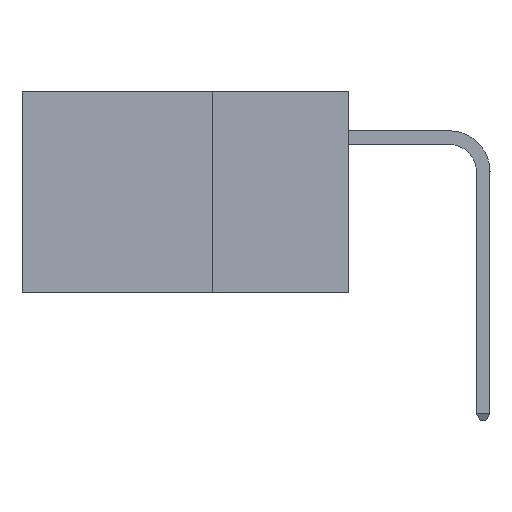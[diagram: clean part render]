
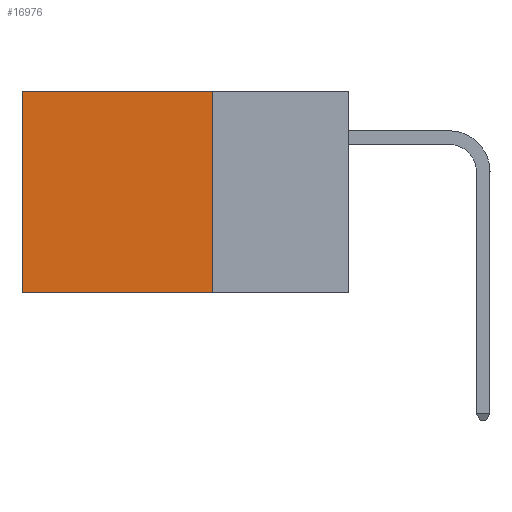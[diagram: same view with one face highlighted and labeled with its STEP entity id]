
A CAD part, left-side view. The second image highlights one B-rep face of the part: STEP entity #16976.
In plain terms, the highlighted planar face has unit normal (-1, 0, 0).
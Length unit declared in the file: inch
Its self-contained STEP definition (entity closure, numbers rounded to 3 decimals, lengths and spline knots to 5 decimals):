
#2449 = EDGE_CURVE ( 'NONE', #22128, #32709, #31265, .T. ) ;
#2577 = CARTESIAN_POINT ( 'NONE',  ( 0.2875, 0.25, 0. ) ) ;
#4612 = CARTESIAN_POINT ( 'NONE',  ( 0.2875, 0.6, 0. ) ) ;
#5254 = DIRECTION ( 'NONE',  ( 0., 0., -1. ) ) ;
#5428 = PLANE ( 'NONE',  #31071 ) ;
#6549 = CARTESIAN_POINT ( 'NONE',  ( 0.2875, 0.6, 0. ) ) ;
#6725 = LINE ( 'NONE', #6549, #17441 ) ;
#6851 = DIRECTION ( 'NONE',  ( 0., 0., -1. ) ) ;
#9070 = DIRECTION ( 'NONE',  ( 0., 1., 0. ) ) ;
#9714 = CARTESIAN_POINT ( 'NONE',  ( 0.2875, 0.25, 0. ) ) ;
#10787 = FACE_OUTER_BOUND ( 'NONE', #27381, .T. ) ;
#10824 = ORIENTED_EDGE ( 'NONE', *, *, #2449, .F. ) ;
#10951 = CARTESIAN_POINT ( 'NONE',  ( 0.2875, 0.25, 0. ) ) ;
#12897 = ORIENTED_EDGE ( 'NONE', *, *, #15180, .T. ) ;
#13443 = DIRECTION ( 'NONE',  ( 1., 0., 0. ) ) ;
#14585 = CARTESIAN_POINT ( 'NONE',  ( 0.2875, 0.25, 0. ) ) ;
#15180 = EDGE_CURVE ( 'NONE', #22128, #31066, #20275, .T. ) ;
#16976 = ADVANCED_FACE ( 'NONE', ( #10787 ), #5428, .F. ) ;
#17441 = VECTOR ( 'NONE', #33453, 39.37008 ) ;
#17581 = VECTOR ( 'NONE', #9070, 39.37008 ) ;
#17589 = CARTESIAN_POINT ( 'NONE',  ( 0.2875, 0.25, -0.37 ) ) ;
#17923 = EDGE_CURVE ( 'NONE', #31066, #30727, #6725, .T. ) ;
#18296 = CARTESIAN_POINT ( 'NONE',  ( 0.2875, 0.25, -0.37 ) ) ;
#20275 = LINE ( 'NONE', #14585, #17581 ) ;
#20780 = VECTOR ( 'NONE', #6851, 39.37008 ) ;
#20958 = ORIENTED_EDGE ( 'NONE', *, *, #32775, .F. ) ;
#21321 = LINE ( 'NONE', #18296, #27883 ) ;
#22128 = VERTEX_POINT ( 'NONE', #10951 ) ;
#24100 = ORIENTED_EDGE ( 'NONE', *, *, #17923, .T. ) ;
#26222 = CARTESIAN_POINT ( 'NONE',  ( 0.2875, 0.6, -0.37 ) ) ;
#27381 = EDGE_LOOP ( 'NONE', ( #24100, #20958, #10824, #12897 ) ) ;
#27883 = VECTOR ( 'NONE', #29161, 39.37008 ) ;
#29161 = DIRECTION ( 'NONE',  ( 0., 1., 0. ) ) ;
#30727 = VERTEX_POINT ( 'NONE', #26222 ) ;
#31066 = VERTEX_POINT ( 'NONE', #4612 ) ;
#31071 = AXIS2_PLACEMENT_3D ( 'NONE', #2577, #13443, #5254 ) ;
#31265 = LINE ( 'NONE', #9714, #20780 ) ;
#32709 = VERTEX_POINT ( 'NONE', #17589 ) ;
#32775 = EDGE_CURVE ( 'NONE', #32709, #30727, #21321, .T. ) ;
#33453 = DIRECTION ( 'NONE',  ( 0., 0., -1. ) ) ;
